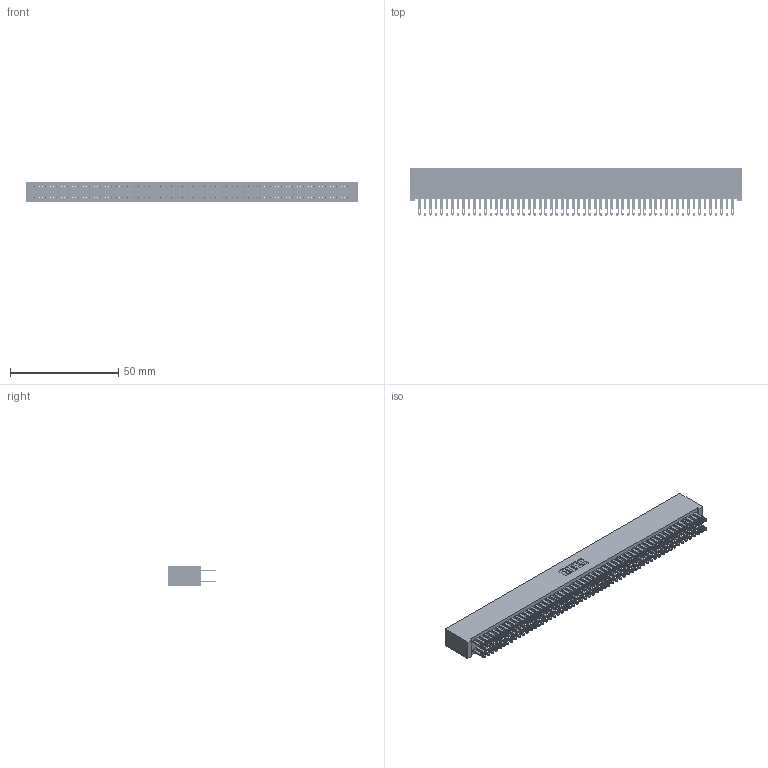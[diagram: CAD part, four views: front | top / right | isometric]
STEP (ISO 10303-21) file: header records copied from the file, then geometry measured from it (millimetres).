
FILE_DESCRIPTION (( 'STEP AP203' ), '1' );
FILE_NAME ('892-116-500-201.STEP', '2020-09-21T22:12:16', ( '' ), ( '' ), 'SwSTEP 2.0', 'SolidWorks 2020', '' );
FILE_SCHEMA (( 'CONFIG_CONTROL_DESIGN' ));
Length unit declared in the file: inch
Products named in the file (3): 842 Part_Lugless; 892-116-500-201; 345-292-001_345-293-100
Assembly tree (117 placements, depth 2):
  892-116-500-201
    842 Part_Lugless
    345-292-001_345-293-100  x116
Bounding box: 153.57 x 21.85 x 9.4 mm (x, y, z)
Volume: 14667.8 mm3; surface area: 25826.6 mm2
Topology: 117 solids, 117 shells, 5670 faces, 17327 edges, 11550 vertices
Faces by surface type: plane 3542, cylinder 2128
Entity records: 34765 total; most frequent: CARTESIAN_POINT 5738, ORIENTED_EDGE 5674, DIRECTION 4869, EDGE_CURVE 2837, VECTOR 2713, LINE 2713, VERTEX_POINT 1890, AXIS2_PLACEMENT_3D 1078
